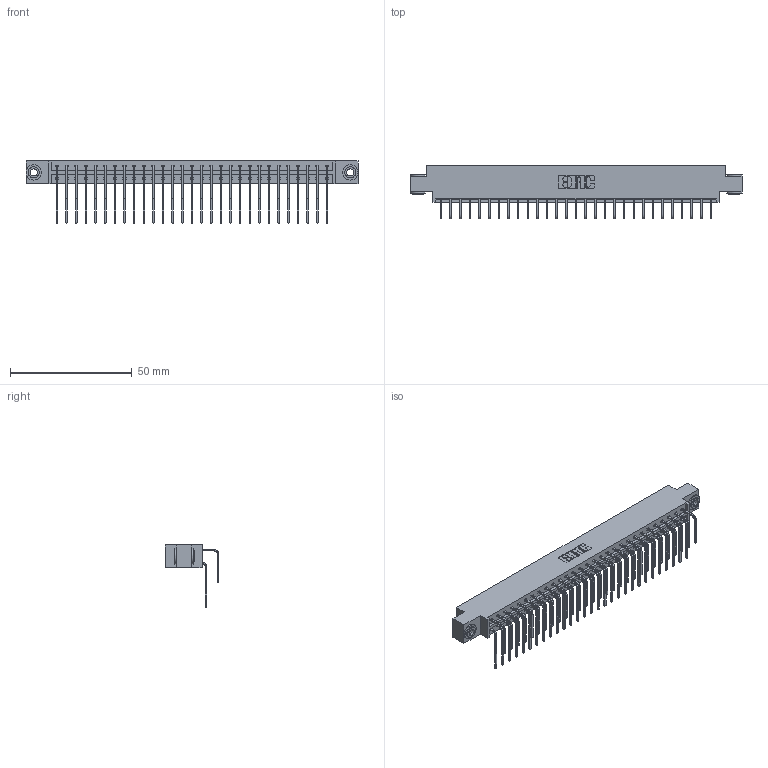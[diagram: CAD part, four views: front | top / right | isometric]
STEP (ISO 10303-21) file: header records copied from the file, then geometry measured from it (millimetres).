
FILE_DESCRIPTION (( 'STEP AP203' ), '1' );
FILE_NAME ('833-058-558-803.STEP', '2020-06-05T01:19:39', ( '' ), ( '' ), 'SwSTEP 2.0', 'SolidWorks 2020', '' );
FILE_SCHEMA (( 'CONFIG_CONTROL_DESIGN' ));
Length unit declared in the file: inch
Products named in the file (5): 345-250-002_345-250-002-102; 833 Part_Offset - .156 Dia - TH; 345-292-001_558 559 Tail - 1; 345-292-001_558 Tail - 2; 833-058-558-803
Assembly tree (61 placements, depth 2):
  833-058-558-803
    833 Part_Offset - .156 Dia - TH
    345-292-001_558 559 Tail - 1  x29
    345-292-001_558 Tail - 2  x29
    345-250-002_345-250-002-102  x2
Bounding box: 136.45 x 22.17 x 25.53 mm (x, y, z)
Volume: 13935.3 mm3; surface area: 18443.6 mm2
Topology: 61 solids, 61 shells, 3288 faces, 9737 edges, 6410 vertices
Faces by surface type: plane 2288, cylinder 992, cone 8
Entity records: 22904 total; most frequent: CARTESIAN_POINT 3840, ORIENTED_EDGE 3718, DIRECTION 3317, EDGE_CURVE 1859, VECTOR 1667, LINE 1667, VERTEX_POINT 1234, AXIS2_PLACEMENT_3D 825
